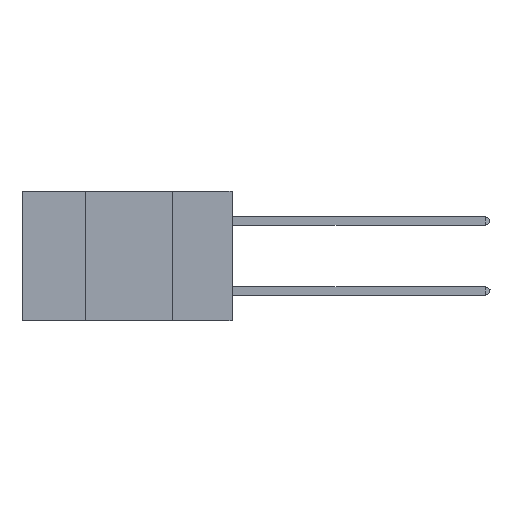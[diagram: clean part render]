
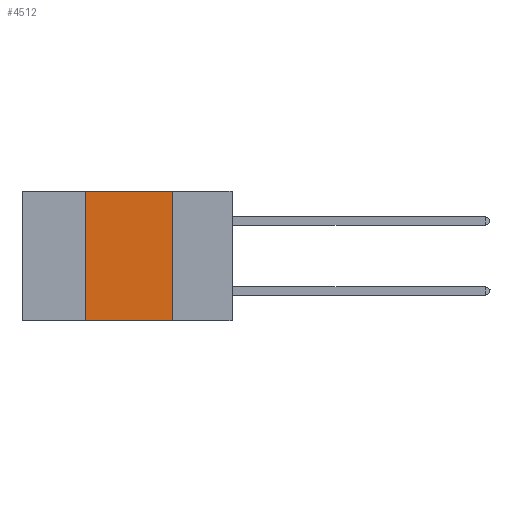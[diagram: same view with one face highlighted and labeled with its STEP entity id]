
A CAD part, left-side view. The second image highlights one B-rep face of the part: STEP entity #4512.
In plain terms, the highlighted planar face has unit normal (-1, 0, 0).
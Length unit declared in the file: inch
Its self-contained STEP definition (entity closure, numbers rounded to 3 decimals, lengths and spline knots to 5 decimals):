
#527 = CARTESIAN_POINT ( 'NONE',  ( 0., 0.42, 0. ) ) ;
#1211 = EDGE_CURVE ( 'NONE', #15514, #17937, #2102, .T. ) ;
#1289 = CARTESIAN_POINT ( 'NONE',  ( 0., 0.42, 0. ) ) ;
#1520 = AXIS2_PLACEMENT_3D ( 'NONE', #12970, #17375, #6326 ) ;
#1525 = ORIENTED_EDGE ( 'NONE', *, *, #3385, .F. ) ;
#1625 = VERTEX_POINT ( 'NONE', #5679 ) ;
#2102 = LINE ( 'NONE', #4785, #4804 ) ;
#2804 = FACE_OUTER_BOUND ( 'NONE', #8121, .T. ) ;
#2877 = LINE ( 'NONE', #527, #17713 ) ;
#2929 = PLANE ( 'NONE',  #1520 ) ;
#3383 = DIRECTION ( 'NONE',  ( 0., 0., -1. ) ) ;
#3385 = EDGE_CURVE ( 'NONE', #10221, #15514, #15367, .T. ) ;
#3996 = ORIENTED_EDGE ( 'NONE', *, *, #8800, .F. ) ;
#4512 = ADVANCED_FACE ( 'NONE', ( #2804 ), #2929, .F. ) ;
#4785 = CARTESIAN_POINT ( 'NONE',  ( 0., 0.17, 0. ) ) ;
#4804 = VECTOR ( 'NONE', #3383, 39.37008 ) ;
#5366 = EDGE_CURVE ( 'NONE', #1625, #17937, #7709, .T. ) ;
#5545 = ORIENTED_EDGE ( 'NONE', *, *, #5366, .T. ) ;
#5679 = CARTESIAN_POINT ( 'NONE',  ( 0., 0.42, -0.37 ) ) ;
#6326 = DIRECTION ( 'NONE',  ( 0., 0., -1. ) ) ;
#6421 = DIRECTION ( 'NONE',  ( 0., 0., 1. ) ) ;
#7187 = DIRECTION ( 'NONE',  ( 0., -1., 0. ) ) ;
#7709 = LINE ( 'NONE', #17398, #12194 ) ;
#8121 = EDGE_LOOP ( 'NONE', ( #15238, #1525, #3996, #5545 ) ) ;
#8800 = EDGE_CURVE ( 'NONE', #1625, #10221, #2877, .T. ) ;
#9757 = CARTESIAN_POINT ( 'NONE',  ( 0., 0.6, 0. ) ) ;
#10221 = VERTEX_POINT ( 'NONE', #1289 ) ;
#10586 = VECTOR ( 'NONE', #7187, 39.37008 ) ;
#12194 = VECTOR ( 'NONE', #16397, 39.37008 ) ;
#12970 = CARTESIAN_POINT ( 'NONE',  ( 0., 0.6, 0. ) ) ;
#13876 = CARTESIAN_POINT ( 'NONE',  ( 0., 0.17, -0.37 ) ) ;
#15238 = ORIENTED_EDGE ( 'NONE', *, *, #1211, .F. ) ;
#15367 = LINE ( 'NONE', #9757, #10586 ) ;
#15514 = VERTEX_POINT ( 'NONE', #18451 ) ;
#16397 = DIRECTION ( 'NONE',  ( 0., -1., 0. ) ) ;
#17375 = DIRECTION ( 'NONE',  ( 1., 0., 0. ) ) ;
#17398 = CARTESIAN_POINT ( 'NONE',  ( 0., 0.6, -0.37 ) ) ;
#17713 = VECTOR ( 'NONE', #6421, 39.37008 ) ;
#17937 = VERTEX_POINT ( 'NONE', #13876 ) ;
#18451 = CARTESIAN_POINT ( 'NONE',  ( 0., 0.17, 0. ) ) ;
